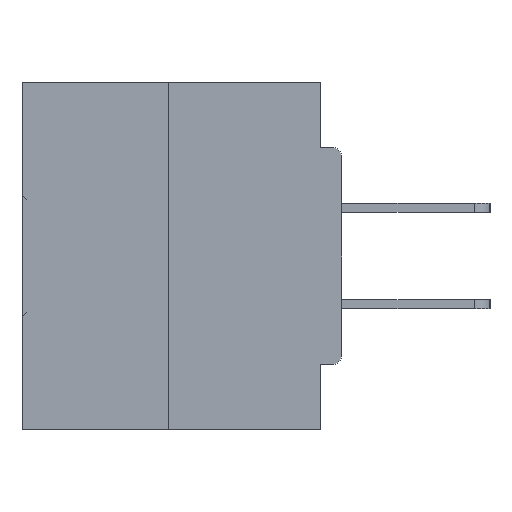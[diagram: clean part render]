
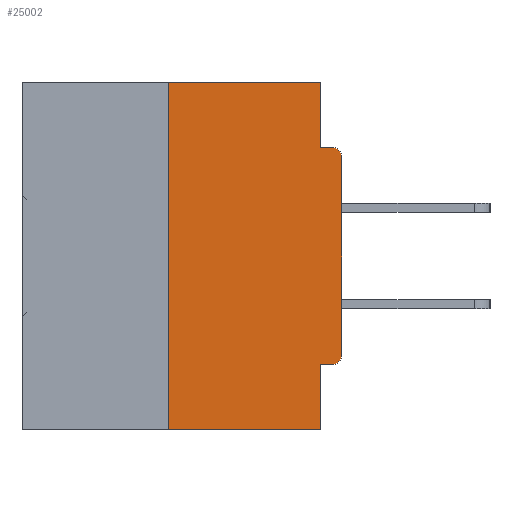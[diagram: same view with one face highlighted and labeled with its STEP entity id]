
A CAD part, left-side view. The second image highlights one B-rep face of the part: STEP entity #25002.
In plain terms, the highlighted planar face has unit normal (-1, 0, 0).
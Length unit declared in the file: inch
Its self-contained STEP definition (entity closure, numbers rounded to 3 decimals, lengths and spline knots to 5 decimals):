
#371 = EDGE_CURVE ( 'NONE', #33576, #15086, #26294, .T. ) ;
#577 = VERTEX_POINT ( 'NONE', #32113 ) ;
#815 = DIRECTION ( 'NONE',  ( 0., -1., 0. ) ) ;
#977 = EDGE_CURVE ( 'NONE', #16279, #16988, #41187, .T. ) ;
#2415 = DIRECTION ( 'NONE',  ( -1., 0., 0. ) ) ;
#2502 = CARTESIAN_POINT ( 'NONE',  ( 0., 0.015, -0.0935 ) ) ;
#2980 = CARTESIAN_POINT ( 'NONE',  ( 0., 0., -0.3915 ) ) ;
#3254 = VERTEX_POINT ( 'NONE', #15985 ) ;
#3337 = PLANE ( 'NONE',  #18165 ) ;
#4697 = CARTESIAN_POINT ( 'NONE',  ( 0., 0.031, 0. ) ) ;
#4891 = DIRECTION ( 'NONE',  ( 0., -1., 0. ) ) ;
#4982 = ORIENTED_EDGE ( 'NONE', *, *, #32472, .T. ) ;
#5456 = VERTEX_POINT ( 'NONE', #22901 ) ;
#7135 = DIRECTION ( 'NONE',  ( 0., -1., 0. ) ) ;
#7957 = ORIENTED_EDGE ( 'NONE', *, *, #977, .F. ) ;
#9703 = VECTOR ( 'NONE', #815, 39.37008 ) ;
#9935 = ORIENTED_EDGE ( 'NONE', *, *, #37641, .T. ) ;
#10786 = LINE ( 'NONE', #15396, #9703 ) ;
#11908 = CIRCLE ( 'NONE', #26339, 0.015 ) ;
#12944 = ORIENTED_EDGE ( 'NONE', *, *, #31278, .F. ) ;
#13910 = LINE ( 'NONE', #21920, #26623 ) ;
#14397 = DIRECTION ( 'NONE',  ( -1., 0., 0. ) ) ;
#14567 = EDGE_CURVE ( 'NONE', #3254, #33280, #43762, .T. ) ;
#15086 = VERTEX_POINT ( 'NONE', #2502 ) ;
#15396 = CARTESIAN_POINT ( 'NONE',  ( 0., 0.46, -0.5 ) ) ;
#15902 = LINE ( 'NONE', #4697, #40276 ) ;
#15985 = CARTESIAN_POINT ( 'NONE',  ( 0., 0.015, -0.4065 ) ) ;
#16279 = VERTEX_POINT ( 'NONE', #21786 ) ;
#16884 = FACE_OUTER_BOUND ( 'NONE', #43334, .T. ) ;
#16988 = VERTEX_POINT ( 'NONE', #29305 ) ;
#17317 = CARTESIAN_POINT ( 'NONE',  ( 0., 0., 0. ) ) ;
#17329 = DIRECTION ( 'NONE',  ( 1., 0., 0. ) ) ;
#17601 = ORIENTED_EDGE ( 'NONE', *, *, #371, .T. ) ;
#17826 = CARTESIAN_POINT ( 'NONE',  ( 0., 0., -0.1085 ) ) ;
#17840 = CARTESIAN_POINT ( 'NONE',  ( 0., 0.25, -0.5 ) ) ;
#18067 = DIRECTION ( 'NONE',  ( 0., 0., 1. ) ) ;
#18165 = AXIS2_PLACEMENT_3D ( 'NONE', #24878, #17329, #35257 ) ;
#18262 = EDGE_CURVE ( 'NONE', #22624, #16279, #30365, .T. ) ;
#18606 = ORIENTED_EDGE ( 'NONE', *, *, #21618, .T. ) ;
#19041 = VECTOR ( 'NONE', #4891, 39.37008 ) ;
#20385 = VECTOR ( 'NONE', #37419, 39.37008 ) ;
#20388 = ORIENTED_EDGE ( 'NONE', *, *, #31035, .F. ) ;
#20465 = AXIS2_PLACEMENT_3D ( 'NONE', #30891, #2415, #44736 ) ;
#21618 = EDGE_CURVE ( 'NONE', #3254, #29743, #11908, .T. ) ;
#21786 = CARTESIAN_POINT ( 'NONE',  ( 0., 0.25, 0. ) ) ;
#21920 = CARTESIAN_POINT ( 'NONE',  ( 0., 0., -0.0935 ) ) ;
#22624 = VERTEX_POINT ( 'NONE', #17840 ) ;
#22901 = CARTESIAN_POINT ( 'NONE',  ( 0., 0.031, -0.0935 ) ) ;
#23336 = CARTESIAN_POINT ( 'NONE',  ( 0., 0.25, 0. ) ) ;
#24878 = CARTESIAN_POINT ( 'NONE',  ( 0., 0.46, 0. ) ) ;
#24901 = ORIENTED_EDGE ( 'NONE', *, *, #14567, .F. ) ;
#25002 = ADVANCED_FACE ( 'NONE', ( #16884 ), #3337, .F. ) ;
#25040 = CARTESIAN_POINT ( 'NONE',  ( 0., 0.015, -0.3915 ) ) ;
#26294 = CIRCLE ( 'NONE', #20465, 0.015 ) ;
#26339 = AXIS2_PLACEMENT_3D ( 'NONE', #25040, #14397, #28746 ) ;
#26623 = VECTOR ( 'NONE', #7135, 39.37008 ) ;
#28746 = DIRECTION ( 'NONE',  ( 0., 0., -1. ) ) ;
#29305 = CARTESIAN_POINT ( 'NONE',  ( 0., 0.031, 0. ) ) ;
#29743 = VERTEX_POINT ( 'NONE', #2980 ) ;
#30365 = LINE ( 'NONE', #23336, #20385 ) ;
#30891 = CARTESIAN_POINT ( 'NONE',  ( 0., 0.015, -0.1085 ) ) ;
#31035 = EDGE_CURVE ( 'NONE', #33280, #577, #32306, .T. ) ;
#31278 = EDGE_CURVE ( 'NONE', #5456, #15086, #13910, .T. ) ;
#32113 = CARTESIAN_POINT ( 'NONE',  ( 0., 0.031, -0.5 ) ) ;
#32306 = LINE ( 'NONE', #45028, #43931 ) ;
#32472 = EDGE_CURVE ( 'NONE', #29743, #33576, #36584, .T. ) ;
#33280 = VERTEX_POINT ( 'NONE', #36461 ) ;
#33576 = VERTEX_POINT ( 'NONE', #17826 ) ;
#34022 = ORIENTED_EDGE ( 'NONE', *, *, #18262, .F. ) ;
#34317 = DIRECTION ( 'NONE',  ( 0., 0., -1. ) ) ;
#35095 = EDGE_CURVE ( 'NONE', #16988, #5456, #15902, .T. ) ;
#35257 = DIRECTION ( 'NONE',  ( 0., 0., -1. ) ) ;
#35993 = VECTOR ( 'NONE', #18067, 39.37008 ) ;
#36077 = CARTESIAN_POINT ( 'NONE',  ( 0., 0.46, 0. ) ) ;
#36461 = CARTESIAN_POINT ( 'NONE',  ( 0., 0.031, -0.4065 ) ) ;
#36573 = VECTOR ( 'NONE', #44624, 39.37008 ) ;
#36584 = LINE ( 'NONE', #17317, #35993 ) ;
#37419 = DIRECTION ( 'NONE',  ( 0., 0., 1. ) ) ;
#37641 = EDGE_CURVE ( 'NONE', #22624, #577, #10786, .T. ) ;
#40276 = VECTOR ( 'NONE', #43154, 39.37008 ) ;
#41187 = LINE ( 'NONE', #36077, #19041 ) ;
#41330 = CARTESIAN_POINT ( 'NONE',  ( 0., 0., -0.4065 ) ) ;
#43154 = DIRECTION ( 'NONE',  ( 0., 0., -1. ) ) ;
#43334 = EDGE_LOOP ( 'NONE', ( #7957, #34022, #9935, #20388, #24901, #18606, #4982, #17601, #12944, #43393 ) ) ;
#43393 = ORIENTED_EDGE ( 'NONE', *, *, #35095, .F. ) ;
#43762 = LINE ( 'NONE', #41330, #36573 ) ;
#43931 = VECTOR ( 'NONE', #34317, 39.37008 ) ;
#44624 = DIRECTION ( 'NONE',  ( 0., 1., 0. ) ) ;
#44736 = DIRECTION ( 'NONE',  ( 0., 0., -1. ) ) ;
#45028 = CARTESIAN_POINT ( 'NONE',  ( 0., 0.031, -0.5 ) ) ;
